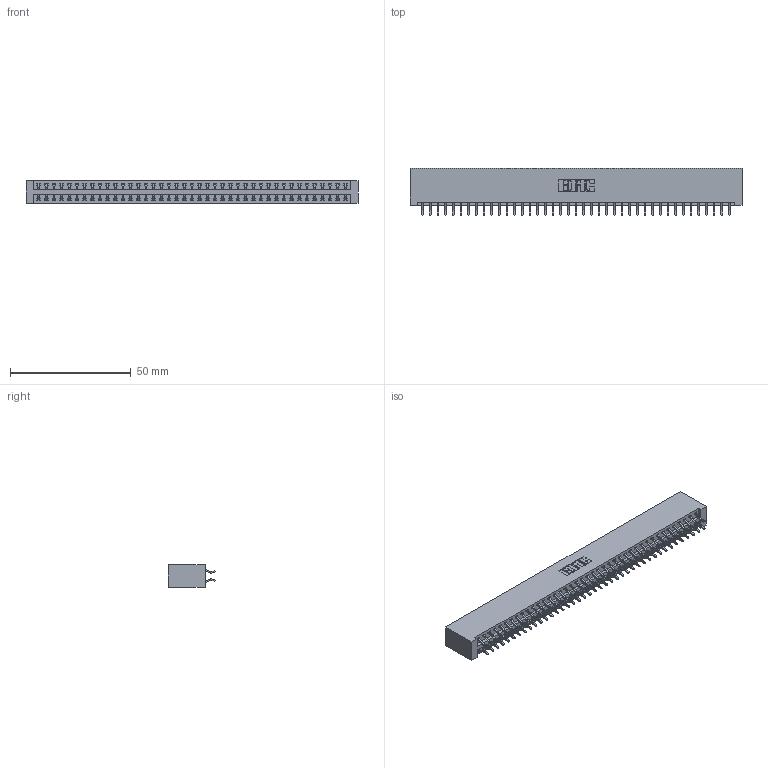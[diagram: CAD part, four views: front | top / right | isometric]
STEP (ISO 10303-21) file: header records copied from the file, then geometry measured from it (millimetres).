
FILE_DESCRIPTION (( 'STEP AP203' ), '1' );
FILE_NAME ('346-082-556-201.STEP', '2022-05-25T18:20:12', ( '' ), ( '' ), 'SwSTEP 2.0', 'SolidWorks 2020', '' );
FILE_SCHEMA (( 'CONFIG_CONTROL_DESIGN' ));
Length unit declared in the file: inch
Products named in the file (3): 346-082-556-201; 346 Part_No Mounting Lugs; 345-292-001_556 Tail
Assembly tree (83 placements, depth 2):
  346-082-556-201
    346 Part_No Mounting Lugs
    345-292-001_556 Tail  x82
Bounding box: 137.41 x 19.57 x 9.4 mm (x, y, z)
Volume: 13961.8 mm3; surface area: 19262.8 mm2
Topology: 83 solids, 83 shells, 4870 faces, 14491 edges, 9550 vertices
Faces by surface type: plane 3270, cylinder 1600
Entity records: 26835 total; most frequent: CARTESIAN_POINT 4436, ORIENTED_EDGE 4358, DIRECTION 3943, EDGE_CURVE 2179, VECTOR 1883, LINE 1883, VERTEX_POINT 1450, AXIS2_PLACEMENT_3D 1030
